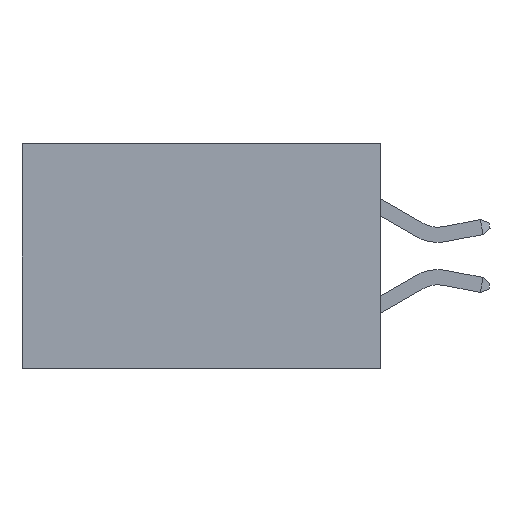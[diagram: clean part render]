
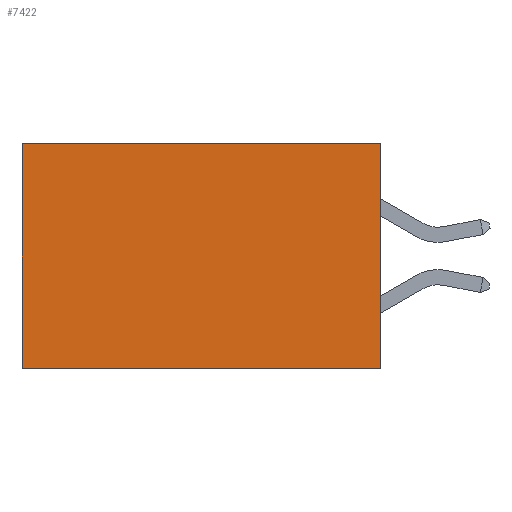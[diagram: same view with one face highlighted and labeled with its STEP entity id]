
A CAD part, left-side view. The second image highlights one B-rep face of the part: STEP entity #7422.
In plain terms, the highlighted planar face has unit normal (-1, 0, 0).
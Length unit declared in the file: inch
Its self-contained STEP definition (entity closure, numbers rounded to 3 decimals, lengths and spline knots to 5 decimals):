
#996 = DIRECTION ( 'NONE',  ( 0., 1., 0. ) ) ;
#1460 = CARTESIAN_POINT ( 'NONE',  ( 0.277, 0., 0. ) ) ;
#2840 = DIRECTION ( 'NONE',  ( 0., 0., -1. ) ) ;
#2876 = DIRECTION ( 'NONE',  ( 1., 0., 0. ) ) ;
#2908 = PLANE ( 'NONE',  #25754 ) ;
#3126 = CARTESIAN_POINT ( 'NONE',  ( 0.277, 0., -0.37 ) ) ;
#3751 = VECTOR ( 'NONE', #996, 39.37008 ) ;
#4469 = CARTESIAN_POINT ( 'NONE',  ( 0.277, 0., 0. ) ) ;
#5755 = ORIENTED_EDGE ( 'NONE', *, *, #7575, .T. ) ;
#5888 = VECTOR ( 'NONE', #16121, 39.37008 ) ;
#5964 = CARTESIAN_POINT ( 'NONE',  ( 0.277, 0., -0.37 ) ) ;
#6711 = VECTOR ( 'NONE', #13402, 39.37008 ) ;
#7422 = ADVANCED_FACE ( 'NONE', ( #19356 ), #2908, .F. ) ;
#7575 = EDGE_CURVE ( 'NONE', #19731, #19085, #21060, .T. ) ;
#9244 = CARTESIAN_POINT ( 'NONE',  ( 0.277, 0.59, 0. ) ) ;
#9771 = EDGE_CURVE ( 'NONE', #19731, #19982, #24015, .T. ) ;
#10484 = ORIENTED_EDGE ( 'NONE', *, *, #15407, .T. ) ;
#12622 = ORIENTED_EDGE ( 'NONE', *, *, #9771, .F. ) ;
#13402 = DIRECTION ( 'NONE',  ( 0., 0., -1. ) ) ;
#14820 = DIRECTION ( 'NONE',  ( 0., 0., -1. ) ) ;
#15407 = EDGE_CURVE ( 'NONE', #19085, #26075, #22887, .T. ) ;
#16121 = DIRECTION ( 'NONE',  ( 0., 1., 0. ) ) ;
#17757 = CARTESIAN_POINT ( 'NONE',  ( 0.277, 0., -0.37 ) ) ;
#18166 = CARTESIAN_POINT ( 'NONE',  ( 0.277, 0.59, -0.37 ) ) ;
#19085 = VERTEX_POINT ( 'NONE', #9244 ) ;
#19356 = FACE_OUTER_BOUND ( 'NONE', #19733, .T. ) ;
#19731 = VERTEX_POINT ( 'NONE', #4469 ) ;
#19733 = EDGE_LOOP ( 'NONE', ( #10484, #23382, #12622, #5755 ) ) ;
#19963 = EDGE_CURVE ( 'NONE', #19982, #26075, #23178, .T. ) ;
#19982 = VERTEX_POINT ( 'NONE', #3126 ) ;
#21060 = LINE ( 'NONE', #1460, #3751 ) ;
#22887 = LINE ( 'NONE', #27607, #27128 ) ;
#23178 = LINE ( 'NONE', #26763, #5888 ) ;
#23382 = ORIENTED_EDGE ( 'NONE', *, *, #19963, .F. ) ;
#24015 = LINE ( 'NONE', #17757, #6711 ) ;
#25754 = AXIS2_PLACEMENT_3D ( 'NONE', #5964, #2876, #2840 ) ;
#26075 = VERTEX_POINT ( 'NONE', #18166 ) ;
#26763 = CARTESIAN_POINT ( 'NONE',  ( 0.277, 0., -0.37 ) ) ;
#27128 = VECTOR ( 'NONE', #14820, 39.37008 ) ;
#27607 = CARTESIAN_POINT ( 'NONE',  ( 0.277, 0.59, -0.37 ) ) ;
